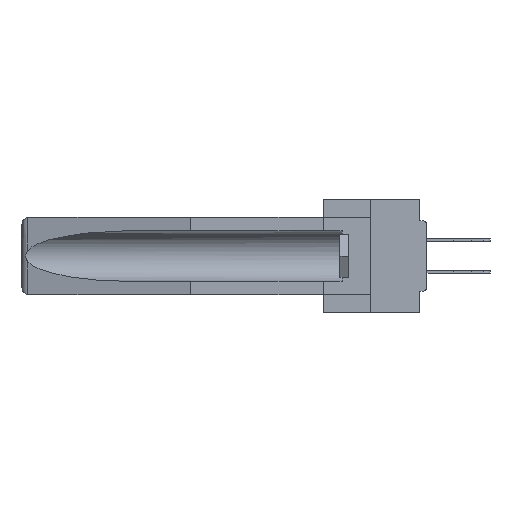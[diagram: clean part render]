
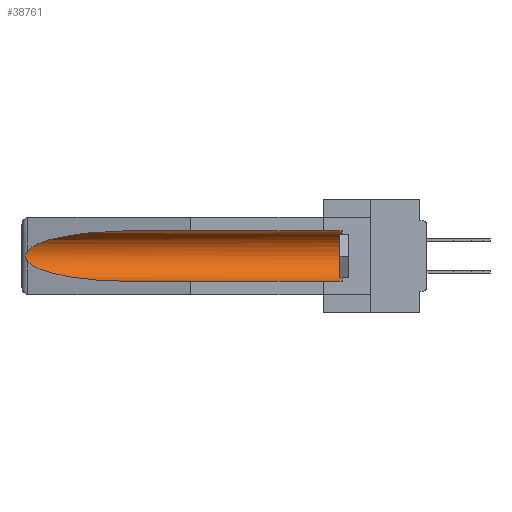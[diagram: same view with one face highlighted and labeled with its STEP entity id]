
A CAD part, left-side view. The second image highlights one B-rep face of the part: STEP entity #38761.
In plain terms, the highlighted cylindrical face has radius 2.857 mm (diameter 5.715 mm), a partial arc.
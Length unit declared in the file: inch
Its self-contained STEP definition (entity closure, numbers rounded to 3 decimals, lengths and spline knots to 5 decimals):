
#1721 = CARTESIAN_POINT ( 'NONE',  ( 0.155, 1.07973, -0.284 ) ) ;
#2351 = CARTESIAN_POINT ( 'NONE',  ( 0.26597, 1.52961, -0.15275 ) ) ;
#2958 = CARTESIAN_POINT ( 'NONE',  ( 0.26537, 1.52718, -0.14972 ) ) ;
#3012 = ORIENTED_EDGE ( 'NONE', *, *, #27661, .F. ) ;
#3357 = ORIENTED_EDGE ( 'NONE', *, *, #29472, .T. ) ;
#3381 =( BOUNDED_CURVE ( )  B_SPLINE_CURVE ( 3, ( #10985, #37894, #28074, #1721 ),
 .UNSPECIFIED., .F., .T. ) 
 B_SPLINE_CURVE_WITH_KNOTS ( ( 4, 4 ),
 ( 0.1948, 1.5708 ),
 .UNSPECIFIED. ) 
 CURVE ( )  GEOMETRIC_REPRESENTATION_ITEM ( )  RATIONAL_B_SPLINE_CURVE ( ( 1., 0.848, 0.848, 1. ) ) 
 REPRESENTATION_ITEM ( '' )  );
#3893 = ORIENTED_EDGE ( 'NONE', *, *, #12883, .T. ) ;
#4028 = ORIENTED_EDGE ( 'NONE', *, *, #4100, .T. ) ;
#4100 = EDGE_CURVE ( 'NONE', #30064, #32340, #22428, .T. ) ;
#4454 = VECTOR ( 'NONE', #38915, 39.37008 ) ;
#6051 = ORIENTED_EDGE ( 'NONE', *, *, #10717, .T. ) ;
#6225 = EDGE_CURVE ( 'NONE', #8847, #11596, #27391, .T. ) ;
#6869 = CARTESIAN_POINT ( 'NONE',  ( 0.155, 0.126, -0.059 ) ) ;
#7768 = CARTESIAN_POINT ( 'NONE',  ( 0.155, 0.126, -0.1715 ) ) ;
#8435 = DIRECTION ( 'NONE',  ( 0., 1., 0. ) ) ;
#8555 =( BOUNDED_CURVE ( )  B_SPLINE_CURVE ( 3, ( #22573, #22288, #31949, #9290 ),
 .UNSPECIFIED., .F., .T. ) 
 B_SPLINE_CURVE_WITH_KNOTS ( ( 4, 4 ),
 ( 4.71239, 6.08839 ),
 .UNSPECIFIED. ) 
 CURVE ( )  GEOMETRIC_REPRESENTATION_ITEM ( )  RATIONAL_B_SPLINE_CURVE ( ( 1., 0.848, 0.848, 1. ) ) 
 REPRESENTATION_ITEM ( '' )  );
#8614 = CARTESIAN_POINT ( 'NONE',  ( 0.26597, 1.5296, -0.19026 ) ) ;
#8847 = VERTEX_POINT ( 'NONE', #40530 ) ;
#8896 = CARTESIAN_POINT ( 'NONE',  ( 0.2675, 1.53308, -0.16763 ) ) ;
#8998 = CARTESIAN_POINT ( 'NONE',  ( 0.155, -0.30754, -0.1715 ) ) ;
#9290 = CARTESIAN_POINT ( 'NONE',  ( 0.26537, 1.52718, -0.14972 ) ) ;
#10717 = EDGE_CURVE ( 'NONE', #25292, #30064, #8555, .T. ) ;
#10985 = CARTESIAN_POINT ( 'NONE',  ( 0.26537, 1.52718, -0.19328 ) ) ;
#11596 = VERTEX_POINT ( 'NONE', #6869 ) ;
#11875 = CARTESIAN_POINT ( 'NONE',  ( 0.26537, 1.52718, -0.19328 ) ) ;
#11908 = CARTESIAN_POINT ( 'NONE',  ( 0.155, -0.30754, -0.284 ) ) ;
#12167 = CARTESIAN_POINT ( 'NONE',  ( 0.2675, 1.53308, -0.17534 ) ) ;
#12603 = AXIS2_PLACEMENT_3D ( 'NONE', #8998, #8435, #41032 ) ;
#12883 = EDGE_CURVE ( 'NONE', #32340, #13365, #3381, .T. ) ;
#13365 = VERTEX_POINT ( 'NONE', #23960 ) ;
#15313 = CARTESIAN_POINT ( 'NONE',  ( 0.2673, 1.53269, -0.17917 ) ) ;
#16072 = LINE ( 'NONE', #42037, #26296 ) ;
#17030 = AXIS2_PLACEMENT_3D ( 'NONE', #7768, #30270, #30564 ) ;
#18877 = CARTESIAN_POINT ( 'NONE',  ( 0.2673, 1.5327, -0.16383 ) ) ;
#22288 = CARTESIAN_POINT ( 'NONE',  ( 0.21114, 1.30732, -0.059 ) ) ;
#22323 = CARTESIAN_POINT ( 'NONE',  ( 0.155, 1.07973, -0.059 ) ) ;
#22428 = B_SPLINE_CURVE_WITH_KNOTS ( 'NONE', 3,
 ( #28432, #2351, #37965, #18877, #8896, #12167, #15313, #38103, #8614, #11875 ),
 .UNSPECIFIED., .F., .F.,
 ( 4, 2, 2, 2, 4 ),
 ( 0., 0.00029, 0.00058, 0.00087, 0.00117 ),
 .UNSPECIFIED. ) ;
#22573 = CARTESIAN_POINT ( 'NONE',  ( 0.155, 1.07973, -0.059 ) ) ;
#23960 = CARTESIAN_POINT ( 'NONE',  ( 0.155, 1.07973, -0.284 ) ) ;
#25292 = VERTEX_POINT ( 'NONE', #22323 ) ;
#26296 = VECTOR ( 'NONE', #29521, 39.37008 ) ;
#27391 = CIRCLE ( 'NONE', #17030, 0.1125 ) ;
#27661 = EDGE_CURVE ( 'NONE', #8847, #13365, #37567, .T. ) ;
#28074 = CARTESIAN_POINT ( 'NONE',  ( 0.21114, 1.30732, -0.284 ) ) ;
#28432 = CARTESIAN_POINT ( 'NONE',  ( 0.26537, 1.52718, -0.14972 ) ) ;
#29472 = EDGE_CURVE ( 'NONE', #11596, #25292, #16072, .T. ) ;
#29521 = DIRECTION ( 'NONE',  ( 0., 1., 0. ) ) ;
#30064 = VERTEX_POINT ( 'NONE', #2958 ) ;
#30270 = DIRECTION ( 'NONE',  ( 0., -1., 0. ) ) ;
#30564 = DIRECTION ( 'NONE',  ( 0., 0., 1. ) ) ;
#31949 = CARTESIAN_POINT ( 'NONE',  ( 0.25451, 1.48313, -0.09465 ) ) ;
#32226 = ORIENTED_EDGE ( 'NONE', *, *, #6225, .T. ) ;
#32340 = VERTEX_POINT ( 'NONE', #33783 ) ;
#33783 = CARTESIAN_POINT ( 'NONE',  ( 0.26537, 1.52718, -0.19328 ) ) ;
#37436 = EDGE_LOOP ( 'NONE', ( #6051, #4028, #3893, #3012, #32226, #3357 ) ) ;
#37567 = LINE ( 'NONE', #11908, #4454 ) ;
#37894 = CARTESIAN_POINT ( 'NONE',  ( 0.25451, 1.48313, -0.24835 ) ) ;
#37965 = CARTESIAN_POINT ( 'NONE',  ( 0.26654, 1.53092, -0.15636 ) ) ;
#38103 = CARTESIAN_POINT ( 'NONE',  ( 0.26655, 1.53094, -0.18657 ) ) ;
#38761 = ADVANCED_FACE ( 'NONE', ( #41992 ), #39749, .F. ) ;
#38915 = DIRECTION ( 'NONE',  ( 0., 1., 0. ) ) ;
#39749 = CYLINDRICAL_SURFACE ( 'NONE', #12603, 0.1125 ) ;
#40530 = CARTESIAN_POINT ( 'NONE',  ( 0.155, 0.126, -0.284 ) ) ;
#41032 = DIRECTION ( 'NONE',  ( 0., 0., 1. ) ) ;
#41992 = FACE_OUTER_BOUND ( 'NONE', #37436, .T. ) ;
#42037 = CARTESIAN_POINT ( 'NONE',  ( 0.155, -0.30754, -0.059 ) ) ;
